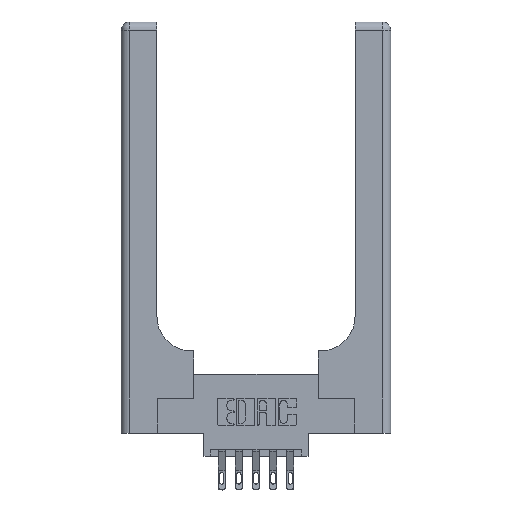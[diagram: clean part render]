
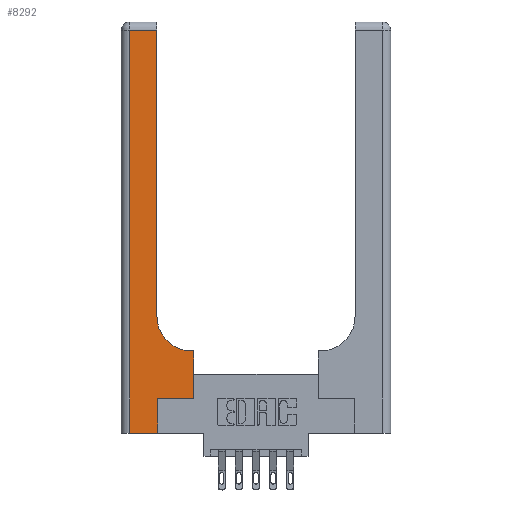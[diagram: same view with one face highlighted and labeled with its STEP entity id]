
A CAD part, top view. The second image highlights one B-rep face of the part: STEP entity #8292.
In plain terms, the highlighted planar face has unit normal (0, 0, 1).
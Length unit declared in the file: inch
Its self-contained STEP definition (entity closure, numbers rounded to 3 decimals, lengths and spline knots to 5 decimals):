
#80 = ORIENTED_EDGE ( 'NONE', *, *, #733, .T. ) ;
#246 = VERTEX_POINT ( 'NONE', #8930 ) ;
#271 = DIRECTION ( 'NONE',  ( 1., 0., 0. ) ) ;
#363 = CARTESIAN_POINT ( 'NONE',  ( 0.528, 0.6, 0.37 ) ) ;
#556 = EDGE_CURVE ( 'NONE', #8015, #6143, #1450, .T. ) ;
#733 = EDGE_CURVE ( 'NONE', #246, #6364, #2980, .T. ) ;
#1027 = CARTESIAN_POINT ( 'NONE',  ( 0.265, 0.25, 0.37 ) ) ;
#1051 = ORIENTED_EDGE ( 'NONE', *, *, #12816, .T. ) ;
#1137 = VECTOR ( 'NONE', #12262, 39.37008 ) ;
#1313 = DIRECTION ( 'NONE',  ( -1., 0., 0. ) ) ;
#1450 = LINE ( 'NONE', #1027, #12530 ) ;
#1455 = VECTOR ( 'NONE', #9272, 39.37008 ) ;
#2192 = CARTESIAN_POINT ( 'NONE',  ( 0.26, 0.6, 0.37 ) ) ;
#2339 = LINE ( 'NONE', #12040, #13419 ) ;
#2349 = CARTESIAN_POINT ( 'NONE',  ( 0.51, 0.6, 0.37 ) ) ;
#2451 = CARTESIAN_POINT ( 'NONE',  ( 0.26, 0.85, 0.37 ) ) ;
#2456 = VERTEX_POINT ( 'NONE', #2349 ) ;
#2458 = CARTESIAN_POINT ( 'NONE',  ( 0.265, 0., 0.37 ) ) ;
#2647 = EDGE_CURVE ( 'NONE', #6143, #12174, #4056, .T. ) ;
#2683 = CARTESIAN_POINT ( 'NONE',  ( 0.528, 0.25, 0.37 ) ) ;
#2980 = LINE ( 'NONE', #12026, #10545 ) ;
#3591 = VERTEX_POINT ( 'NONE', #2458 ) ;
#3681 = ORIENTED_EDGE ( 'NONE', *, *, #2647, .T. ) ;
#4056 = LINE ( 'NONE', #2683, #1137 ) ;
#4581 = DIRECTION ( 'NONE',  ( 0., -1., 0. ) ) ;
#5427 = VERTEX_POINT ( 'NONE', #7918 ) ;
#5438 = CARTESIAN_POINT ( 'NONE',  ( 0.06, 2.94, 0.37 ) ) ;
#5483 = VECTOR ( 'NONE', #12997, 39.37008 ) ;
#6109 = PLANE ( 'NONE',  #12449 ) ;
#6143 = VERTEX_POINT ( 'NONE', #12511 ) ;
#6181 = ORIENTED_EDGE ( 'NONE', *, *, #11009, .T. ) ;
#6364 = VERTEX_POINT ( 'NONE', #5438 ) ;
#6755 = DIRECTION ( 'NONE',  ( 0., 0., -1. ) ) ;
#6990 = EDGE_CURVE ( 'NONE', #3591, #8015, #8328, .T. ) ;
#7177 = DIRECTION ( 'NONE',  ( -1., 0., 0. ) ) ;
#7234 = LINE ( 'NONE', #13497, #1455 ) ;
#7465 = AXIS2_PLACEMENT_3D ( 'NONE', #13112, #6755, #271 ) ;
#7489 = EDGE_LOOP ( 'NONE', ( #13802, #80, #6181, #1051, #9559, #7517, #3681, #11861, #11654 ) ) ;
#7517 = ORIENTED_EDGE ( 'NONE', *, *, #556, .T. ) ;
#7918 = CARTESIAN_POINT ( 'NONE',  ( 0.06, 0., 0.37 ) ) ;
#7957 = CARTESIAN_POINT ( 'NONE',  ( 0., 0., 0.37 ) ) ;
#8015 = VERTEX_POINT ( 'NONE', #8661 ) ;
#8292 = ADVANCED_FACE ( 'NONE', ( #13780 ), #6109, .F. ) ;
#8328 = LINE ( 'NONE', #9757, #5483 ) ;
#8648 = DIRECTION ( 'NONE',  ( -1., 0., 0. ) ) ;
#8661 = CARTESIAN_POINT ( 'NONE',  ( 0.265, 0.25, 0.37 ) ) ;
#8716 = VECTOR ( 'NONE', #8648, 39.37008 ) ;
#8930 = CARTESIAN_POINT ( 'NONE',  ( 0.26, 2.94, 0.37 ) ) ;
#9014 = DIRECTION ( 'NONE',  ( 1., 0., 0. ) ) ;
#9272 = DIRECTION ( 'NONE',  ( 0., 1., 0. ) ) ;
#9559 = ORIENTED_EDGE ( 'NONE', *, *, #6990, .T. ) ;
#9757 = CARTESIAN_POINT ( 'NONE',  ( 0.265, 0., 0.37 ) ) ;
#10339 = CARTESIAN_POINT ( 'NONE',  ( 0., 3., 0.37 ) ) ;
#10381 = VECTOR ( 'NONE', #9014, 39.37008 ) ;
#10545 = VECTOR ( 'NONE', #1313, 39.37008 ) ;
#10920 = CIRCLE ( 'NONE', #7465, 0.25 ) ;
#11002 = EDGE_CURVE ( 'NONE', #2456, #13321, #10920, .T. ) ;
#11009 = EDGE_CURVE ( 'NONE', #6364, #5427, #2339, .T. ) ;
#11654 = ORIENTED_EDGE ( 'NONE', *, *, #11002, .T. ) ;
#11861 = ORIENTED_EDGE ( 'NONE', *, *, #12575, .T. ) ;
#12026 = CARTESIAN_POINT ( 'NONE',  ( 0., 2.94, 0.37 ) ) ;
#12040 = CARTESIAN_POINT ( 'NONE',  ( 0.06, 3., 0.37 ) ) ;
#12174 = VERTEX_POINT ( 'NONE', #363 ) ;
#12262 = DIRECTION ( 'NONE',  ( 0., 1., 0. ) ) ;
#12391 = EDGE_CURVE ( 'NONE', #13321, #246, #7234, .T. ) ;
#12449 = AXIS2_PLACEMENT_3D ( 'NONE', #10339, #13559, #7177 ) ;
#12511 = CARTESIAN_POINT ( 'NONE',  ( 0.528, 0.25, 0.37 ) ) ;
#12530 = VECTOR ( 'NONE', #13902, 39.37008 ) ;
#12575 = EDGE_CURVE ( 'NONE', #12174, #2456, #13380, .T. ) ;
#12816 = EDGE_CURVE ( 'NONE', #5427, #3591, #13211, .T. ) ;
#12997 = DIRECTION ( 'NONE',  ( 0., 1., 0. ) ) ;
#13112 = CARTESIAN_POINT ( 'NONE',  ( 0.51, 0.85, 0.37 ) ) ;
#13211 = LINE ( 'NONE', #7957, #10381 ) ;
#13321 = VERTEX_POINT ( 'NONE', #2451 ) ;
#13380 = LINE ( 'NONE', #2192, #8716 ) ;
#13419 = VECTOR ( 'NONE', #4581, 39.37008 ) ;
#13497 = CARTESIAN_POINT ( 'NONE',  ( 0.26, 3., 0.37 ) ) ;
#13559 = DIRECTION ( 'NONE',  ( 0., 0., -1. ) ) ;
#13780 = FACE_OUTER_BOUND ( 'NONE', #7489, .T. ) ;
#13802 = ORIENTED_EDGE ( 'NONE', *, *, #12391, .T. ) ;
#13902 = DIRECTION ( 'NONE',  ( 1., 0., 0. ) ) ;
